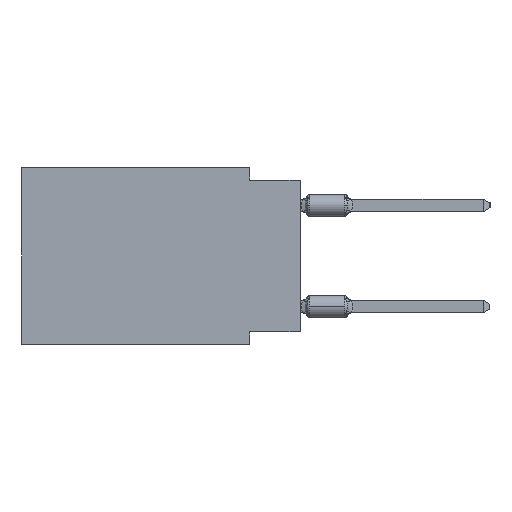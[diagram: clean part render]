
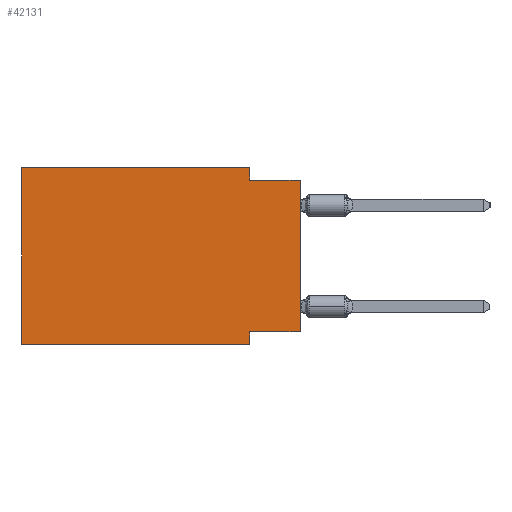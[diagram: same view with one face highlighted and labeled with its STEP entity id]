
A CAD part, left-side view. The second image highlights one B-rep face of the part: STEP entity #42131.
In plain terms, the highlighted planar face has unit normal (-1, 0, 0).
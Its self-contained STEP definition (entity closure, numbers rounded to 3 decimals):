
#470 = CARTESIAN_POINT ( 'NONE',  ( 0., 0., -0.635 ) ) ;
#1975 = EDGE_LOOP ( 'NONE', ( #9422, #24958, #17275, #28238, #48487, #33577, #10560, #16263 ) ) ;
#4531 = CARTESIAN_POINT ( 'NONE',  ( 0., 2.54, -0.635 ) ) ;
#4705 = LINE ( 'NONE', #26270, #33562 ) ;
#6269 = CARTESIAN_POINT ( 'NONE',  ( 0., 13.97, -8.89 ) ) ;
#7363 = VECTOR ( 'NONE', #19136, 1000. ) ;
#8361 = LINE ( 'NONE', #47445, #15588 ) ;
#9422 = ORIENTED_EDGE ( 'NONE', *, *, #51911, .T. ) ;
#10136 = LINE ( 'NONE', #19327, #25447 ) ;
#10152 = CARTESIAN_POINT ( 'NONE',  ( 0., 13.97, -8.89 ) ) ;
#10560 = ORIENTED_EDGE ( 'NONE', *, *, #51769, .F. ) ;
#11663 = EDGE_CURVE ( 'NONE', #12012, #49398, #8361, .T. ) ;
#12012 = VERTEX_POINT ( 'NONE', #46805 ) ;
#13259 = CARTESIAN_POINT ( 'NONE',  ( 0., 2.54, 0. ) ) ;
#14171 = PLANE ( 'NONE',  #43434 ) ;
#14712 = LINE ( 'NONE', #54032, #48897 ) ;
#15588 = VECTOR ( 'NONE', #43126, 1000. ) ;
#16263 = ORIENTED_EDGE ( 'NONE', *, *, #56775, .F. ) ;
#16591 = DIRECTION ( 'NONE',  ( 0., -1., 0. ) ) ;
#16675 = EDGE_CURVE ( 'NONE', #49398, #27159, #10136, .T. ) ;
#17275 = ORIENTED_EDGE ( 'NONE', *, *, #16675, .F. ) ;
#18286 = LINE ( 'NONE', #470, #7363 ) ;
#18492 = VERTEX_POINT ( 'NONE', #43971 ) ;
#18942 = EDGE_CURVE ( 'NONE', #27159, #18492, #18286, .T. ) ;
#19136 = DIRECTION ( 'NONE',  ( 0., -1., 0. ) ) ;
#19327 = CARTESIAN_POINT ( 'NONE',  ( 0., 2.54, 0. ) ) ;
#19775 = VERTEX_POINT ( 'NONE', #43711 ) ;
#20799 = CARTESIAN_POINT ( 'NONE',  ( 0., 2.54, -8.255 ) ) ;
#22785 = FACE_OUTER_BOUND ( 'NONE', #1975, .T. ) ;
#23064 = CARTESIAN_POINT ( 'NONE',  ( 0., 13.97, 0. ) ) ;
#23942 = LINE ( 'NONE', #41167, #31724 ) ;
#24958 = ORIENTED_EDGE ( 'NONE', *, *, #18942, .F. ) ;
#25447 = VECTOR ( 'NONE', #28507, 1000. ) ;
#26270 = CARTESIAN_POINT ( 'NONE',  ( 0., 2.54, -8.89 ) ) ;
#27159 = VERTEX_POINT ( 'NONE', #4531 ) ;
#28117 = LINE ( 'NONE', #6269, #28930 ) ;
#28238 = ORIENTED_EDGE ( 'NONE', *, *, #11663, .F. ) ;
#28507 = DIRECTION ( 'NONE',  ( 0., 0., -1. ) ) ;
#28930 = VECTOR ( 'NONE', #16591, 1000. ) ;
#31267 = CARTESIAN_POINT ( 'NONE',  ( 0., 0., -8.255 ) ) ;
#31724 = VECTOR ( 'NONE', #36584, 1000. ) ;
#32233 = DIRECTION ( 'NONE',  ( 0., 0., 1. ) ) ;
#33562 = VECTOR ( 'NONE', #52659, 1000. ) ;
#33577 = ORIENTED_EDGE ( 'NONE', *, *, #51169, .T. ) ;
#33613 = VECTOR ( 'NONE', #56532, 1000. ) ;
#36584 = DIRECTION ( 'NONE',  ( 0., 0., 1. ) ) ;
#37081 = VERTEX_POINT ( 'NONE', #20799 ) ;
#38921 = VERTEX_POINT ( 'NONE', #10152 ) ;
#40611 = VERTEX_POINT ( 'NONE', #44317 ) ;
#41167 = CARTESIAN_POINT ( 'NONE',  ( 0., 0., 0. ) ) ;
#42131 = ADVANCED_FACE ( 'NONE', ( #22785 ), #14171, .F. ) ;
#43126 = DIRECTION ( 'NONE',  ( 0., -1., 0. ) ) ;
#43434 = AXIS2_PLACEMENT_3D ( 'NONE', #23064, #44037, #44611 ) ;
#43711 = CARTESIAN_POINT ( 'NONE',  ( 0., 0., -8.255 ) ) ;
#43908 = LINE ( 'NONE', #31267, #33613 ) ;
#43971 = CARTESIAN_POINT ( 'NONE',  ( 0., 0., -0.635 ) ) ;
#44037 = DIRECTION ( 'NONE',  ( 1., 0., 0. ) ) ;
#44317 = CARTESIAN_POINT ( 'NONE',  ( 0., 2.54, -8.89 ) ) ;
#44611 = DIRECTION ( 'NONE',  ( 0., 0., -1. ) ) ;
#46805 = CARTESIAN_POINT ( 'NONE',  ( 0., 13.97, 0. ) ) ;
#47445 = CARTESIAN_POINT ( 'NONE',  ( 0., 13.97, 0. ) ) ;
#48487 = ORIENTED_EDGE ( 'NONE', *, *, #53522, .F. ) ;
#48897 = VECTOR ( 'NONE', #32233, 1000. ) ;
#49398 = VERTEX_POINT ( 'NONE', #13259 ) ;
#51169 = EDGE_CURVE ( 'NONE', #38921, #40611, #28117, .T. ) ;
#51769 = EDGE_CURVE ( 'NONE', #37081, #40611, #4705, .T. ) ;
#51911 = EDGE_CURVE ( 'NONE', #19775, #18492, #23942, .T. ) ;
#52659 = DIRECTION ( 'NONE',  ( 0., 0., -1. ) ) ;
#53522 = EDGE_CURVE ( 'NONE', #38921, #12012, #14712, .T. ) ;
#54032 = CARTESIAN_POINT ( 'NONE',  ( 0., 13.97, 0. ) ) ;
#56532 = DIRECTION ( 'NONE',  ( 0., 1., 0. ) ) ;
#56775 = EDGE_CURVE ( 'NONE', #19775, #37081, #43908, .T. ) ;
